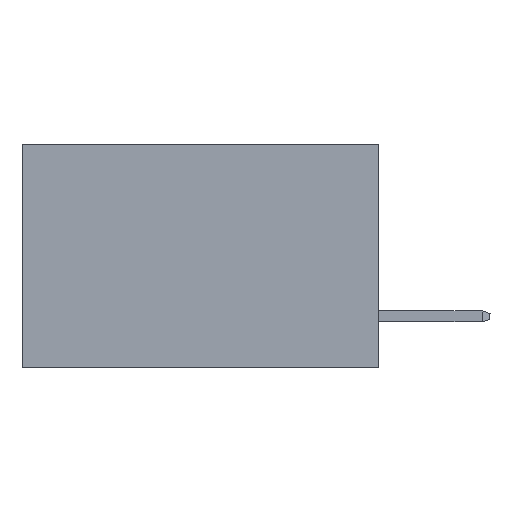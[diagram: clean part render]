
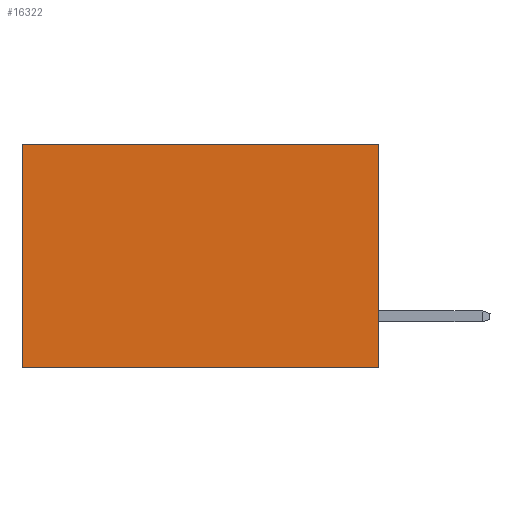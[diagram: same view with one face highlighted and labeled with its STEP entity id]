
A CAD part, left-side view. The second image highlights one B-rep face of the part: STEP entity #16322.
In plain terms, the highlighted planar face has unit normal (-1, 0, 0).
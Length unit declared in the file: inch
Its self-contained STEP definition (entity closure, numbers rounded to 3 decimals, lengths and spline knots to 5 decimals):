
#1446 = LINE ( 'NONE', #27612, #7397 ) ;
#5116 = EDGE_CURVE ( 'NONE', #11696, #8602, #1446, .T. ) ;
#6261 = CARTESIAN_POINT ( 'NONE',  ( 0.277, 0., -0.37 ) ) ;
#7397 = VECTOR ( 'NONE', #20766, 39.37008 ) ;
#7978 = CARTESIAN_POINT ( 'NONE',  ( 0.277, 0., -0.37 ) ) ;
#8310 = DIRECTION ( 'NONE',  ( 0., 0., -1. ) ) ;
#8602 = VERTEX_POINT ( 'NONE', #25078 ) ;
#8660 = DIRECTION ( 'NONE',  ( 0., 1., 0. ) ) ;
#8871 = VECTOR ( 'NONE', #8660, 39.37008 ) ;
#9205 = AXIS2_PLACEMENT_3D ( 'NONE', #7978, #10243, #26098 ) ;
#9398 = DIRECTION ( 'NONE',  ( 0., 1., 0. ) ) ;
#10243 = DIRECTION ( 'NONE',  ( 1., 0., 0. ) ) ;
#10841 = ORIENTED_EDGE ( 'NONE', *, *, #18573, .T. ) ;
#11696 = VERTEX_POINT ( 'NONE', #23630 ) ;
#12447 = EDGE_LOOP ( 'NONE', ( #19215, #26060, #18144, #10841 ) ) ;
#13413 = LINE ( 'NONE', #13841, #19369 ) ;
#13823 = FACE_OUTER_BOUND ( 'NONE', #12447, .T. ) ;
#13841 = CARTESIAN_POINT ( 'NONE',  ( 0.277, 0., -0.37 ) ) ;
#14197 = CARTESIAN_POINT ( 'NONE',  ( 0.277, 0., 0. ) ) ;
#16322 = ADVANCED_FACE ( 'NONE', ( #13823 ), #21502, .F. ) ;
#17115 = VERTEX_POINT ( 'NONE', #6261 ) ;
#18144 = ORIENTED_EDGE ( 'NONE', *, *, #28572, .F. ) ;
#18573 = EDGE_CURVE ( 'NONE', #23877, #11696, #21599, .T. ) ;
#19215 = ORIENTED_EDGE ( 'NONE', *, *, #5116, .T. ) ;
#19369 = VECTOR ( 'NONE', #9398, 39.37008 ) ;
#20766 = DIRECTION ( 'NONE',  ( 0., 0., -1. ) ) ;
#21502 = PLANE ( 'NONE',  #9205 ) ;
#21599 = LINE ( 'NONE', #29005, #8871 ) ;
#22644 = LINE ( 'NONE', #24186, #27906 ) ;
#23630 = CARTESIAN_POINT ( 'NONE',  ( 0.277, 0.59, 0. ) ) ;
#23877 = VERTEX_POINT ( 'NONE', #14197 ) ;
#24186 = CARTESIAN_POINT ( 'NONE',  ( 0.277, 0., -0.37 ) ) ;
#25078 = CARTESIAN_POINT ( 'NONE',  ( 0.277, 0.59, -0.37 ) ) ;
#26060 = ORIENTED_EDGE ( 'NONE', *, *, #28899, .F. ) ;
#26098 = DIRECTION ( 'NONE',  ( 0., 0., -1. ) ) ;
#27612 = CARTESIAN_POINT ( 'NONE',  ( 0.277, 0.59, -0.37 ) ) ;
#27906 = VECTOR ( 'NONE', #8310, 39.37008 ) ;
#28572 = EDGE_CURVE ( 'NONE', #23877, #17115, #22644, .T. ) ;
#28899 = EDGE_CURVE ( 'NONE', #17115, #8602, #13413, .T. ) ;
#29005 = CARTESIAN_POINT ( 'NONE',  ( 0.277, 0., 0. ) ) ;
